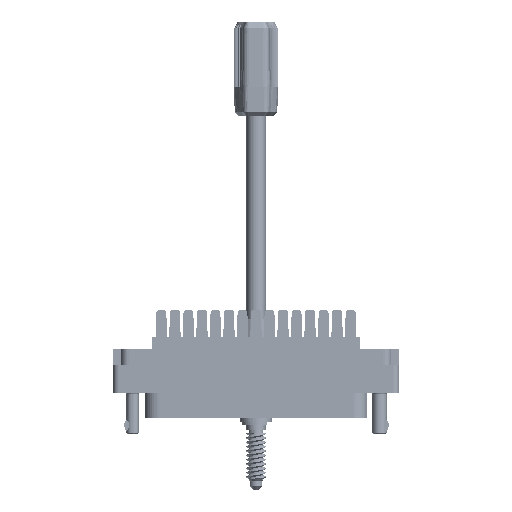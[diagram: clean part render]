
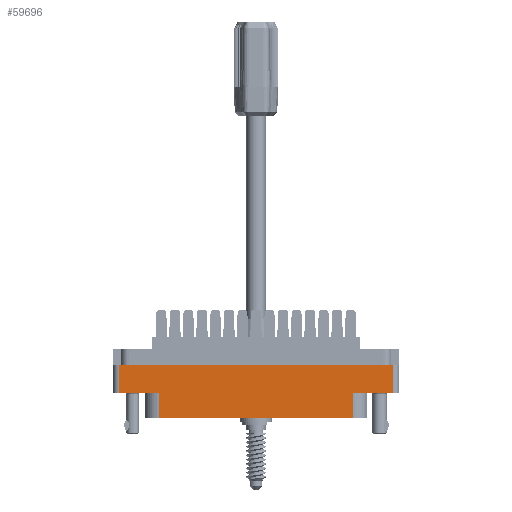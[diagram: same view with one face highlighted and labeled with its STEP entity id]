
A CAD part, front view. The second image highlights one B-rep face of the part: STEP entity #59696.
In plain terms, the highlighted planar face has unit normal (0, -1, 0).
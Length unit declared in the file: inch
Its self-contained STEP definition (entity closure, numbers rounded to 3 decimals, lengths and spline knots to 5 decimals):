
#139 = LINE ( 'NONE', #41522, #54304 ) ;
#1464 = DIRECTION ( 'NONE',  ( 0., 0., 1. ) ) ;
#4133 = EDGE_CURVE ( 'NONE', #23829, #40386, #111342, .T. ) ;
#4415 = CARTESIAN_POINT ( 'NONE',  ( 1.313, -0.7625, -0.274 ) ) ;
#5905 = CARTESIAN_POINT ( 'NONE',  ( -0.9315, -0.7625, -0.78 ) ) ;
#6245 = DIRECTION ( 'NONE',  ( 1., 0., 0. ) ) ;
#7032 = LINE ( 'NONE', #5905, #73067 ) ;
#8406 = DIRECTION ( 'NONE',  ( 0., 0., -1. ) ) ;
#8986 = DIRECTION ( 'NONE',  ( 0., -1., 0. ) ) ;
#9757 = CARTESIAN_POINT ( 'NONE',  ( -1.313, -0.7625, -0.274 ) ) ;
#9961 = DIRECTION ( 'NONE',  ( -1., 0., 0. ) ) ;
#10173 = VECTOR ( 'NONE', #70719, 39.37008 ) ;
#12107 = CARTESIAN_POINT ( 'NONE',  ( -1.313, -0.7625, -0.54 ) ) ;
#12820 = ORIENTED_EDGE ( 'NONE', *, *, #75789, .T. ) ;
#14877 = CARTESIAN_POINT ( 'NONE',  ( -1.375, -0.7625, -0.78 ) ) ;
#16365 = ORIENTED_EDGE ( 'NONE', *, *, #39412, .T. ) ;
#17504 = LINE ( 'NONE', #50274, #39936 ) ;
#19876 = ORIENTED_EDGE ( 'NONE', *, *, #85979, .F. ) ;
#22663 = VERTEX_POINT ( 'NONE', #56263 ) ;
#23829 = VERTEX_POINT ( 'NONE', #97281 ) ;
#24679 = LINE ( 'NONE', #68883, #113226 ) ;
#25371 = CARTESIAN_POINT ( 'NONE',  ( -1.313, -0.7625, -0.78 ) ) ;
#26554 = DIRECTION ( 'NONE',  ( 1., 0., 0. ) ) ;
#29443 = CARTESIAN_POINT ( 'NONE',  ( 1.313, -0.7625, -0.54 ) ) ;
#31149 = ORIENTED_EDGE ( 'NONE', *, *, #65982, .T. ) ;
#32962 = CARTESIAN_POINT ( 'NONE',  ( 0.9315, -0.7625, -0.54 ) ) ;
#33809 = VECTOR ( 'NONE', #9961, 39.37008 ) ;
#34235 = FACE_OUTER_BOUND ( 'NONE', #89996, .T. ) ;
#35265 = LINE ( 'NONE', #70259, #33809 ) ;
#35628 = VERTEX_POINT ( 'NONE', #4415 ) ;
#35911 = CARTESIAN_POINT ( 'NONE',  ( 0.9315, -0.7625, -0.78 ) ) ;
#38725 = ORIENTED_EDGE ( 'NONE', *, *, #4133, .T. ) ;
#39412 = EDGE_CURVE ( 'NONE', #22663, #23829, #7032, .T. ) ;
#39936 = VECTOR ( 'NONE', #113435, 39.37008 ) ;
#40386 = VERTEX_POINT ( 'NONE', #35911 ) ;
#41522 = CARTESIAN_POINT ( 'NONE',  ( 0., -0.7625, -0.274 ) ) ;
#43921 = VERTEX_POINT ( 'NONE', #9757 ) ;
#44497 = VECTOR ( 'NONE', #6245, 39.37008 ) ;
#46831 = LINE ( 'NONE', #72110, #106663 ) ;
#50274 = CARTESIAN_POINT ( 'NONE',  ( 0., -0.7625, -0.54 ) ) ;
#54304 = VECTOR ( 'NONE', #26554, 39.37008 ) ;
#55500 = ORIENTED_EDGE ( 'NONE', *, *, #101443, .F. ) ;
#56263 = CARTESIAN_POINT ( 'NONE',  ( -0.9315, -0.7625, -0.54 ) ) ;
#59296 = DIRECTION ( 'NONE',  ( 0., 0., -1. ) ) ;
#59696 = ADVANCED_FACE ( 'NONE', ( #34235 ), #70407, .T. ) ;
#61844 = EDGE_CURVE ( 'NONE', #43921, #74920, #87987, .T. ) ;
#62832 = ORIENTED_EDGE ( 'NONE', *, *, #61844, .T. ) ;
#65982 = EDGE_CURVE ( 'NONE', #86091, #35628, #24679, .T. ) ;
#68883 = CARTESIAN_POINT ( 'NONE',  ( 1.313, -0.7625, -0.78 ) ) ;
#70259 = CARTESIAN_POINT ( 'NONE',  ( 0., -0.7625, -0.54 ) ) ;
#70407 = PLANE ( 'NONE',  #88735 ) ;
#70719 = DIRECTION ( 'NONE',  ( 0., 0., -1. ) ) ;
#72110 = CARTESIAN_POINT ( 'NONE',  ( 0.9315, -0.7625, -0.54 ) ) ;
#73067 = VECTOR ( 'NONE', #59296, 39.37008 ) ;
#74920 = VERTEX_POINT ( 'NONE', #12107 ) ;
#75789 = EDGE_CURVE ( 'NONE', #40386, #81777, #46831, .T. ) ;
#81777 = VERTEX_POINT ( 'NONE', #32962 ) ;
#85979 = EDGE_CURVE ( 'NONE', #86091, #81777, #35265, .T. ) ;
#86091 = VERTEX_POINT ( 'NONE', #29443 ) ;
#87987 = LINE ( 'NONE', #25371, #10173 ) ;
#88735 = AXIS2_PLACEMENT_3D ( 'NONE', #106043, #8986, #8406 ) ;
#89996 = EDGE_LOOP ( 'NONE', ( #55500, #62832, #105512, #16365, #38725, #12820, #19876, #31149 ) ) ;
#91660 = EDGE_CURVE ( 'NONE', #74920, #22663, #17504, .T. ) ;
#95917 = DIRECTION ( 'NONE',  ( 0., 0., 1. ) ) ;
#97281 = CARTESIAN_POINT ( 'NONE',  ( -0.9315, -0.7625, -0.78 ) ) ;
#101443 = EDGE_CURVE ( 'NONE', #43921, #35628, #139, .T. ) ;
#105512 = ORIENTED_EDGE ( 'NONE', *, *, #91660, .T. ) ;
#106043 = CARTESIAN_POINT ( 'NONE',  ( -1.375, -0.7625, -0.78 ) ) ;
#106663 = VECTOR ( 'NONE', #1464, 39.37008 ) ;
#111342 = LINE ( 'NONE', #14877, #44497 ) ;
#113226 = VECTOR ( 'NONE', #95917, 39.37008 ) ;
#113435 = DIRECTION ( 'NONE',  ( 1., 0., 0. ) ) ;
